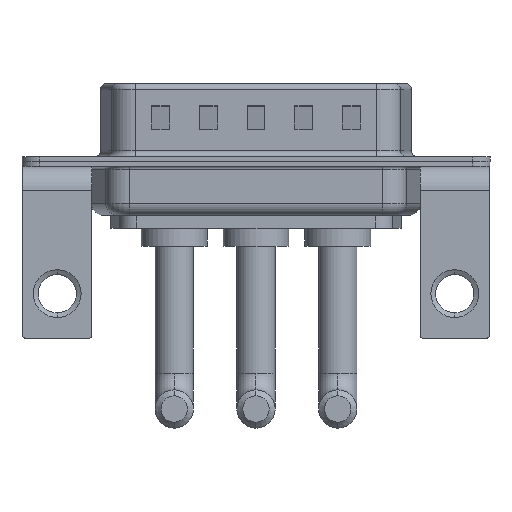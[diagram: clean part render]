
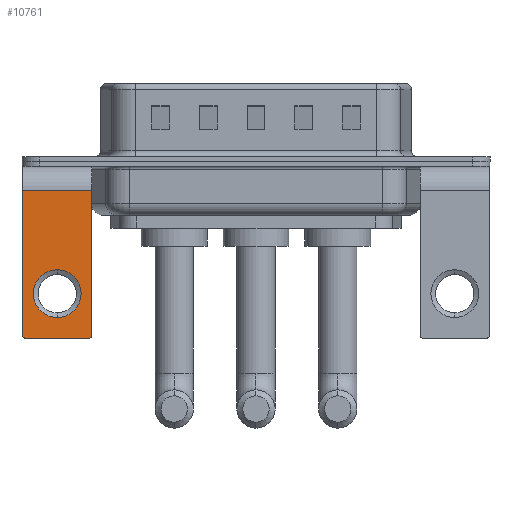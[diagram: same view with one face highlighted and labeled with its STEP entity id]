
A CAD part, front view. The second image highlights one B-rep face of the part: STEP entity #10761.
In plain terms, the highlighted planar face has unit normal (0, -1, 0).
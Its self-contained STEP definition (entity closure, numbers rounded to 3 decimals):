
#5 = DIRECTION ( 'NONE',  ( 0., -1., 0. ) ) ;
#497 = ORIENTED_EDGE ( 'NONE', *, *, #15092, .T. ) ;
#1039 = VERTEX_POINT ( 'NONE', #6492 ) ;
#1051 = VERTEX_POINT ( 'NONE', #1114 ) ;
#1114 = CARTESIAN_POINT ( 'NONE',  ( 2.65, -6.25, -14.8 ) ) ;
#1489 = LINE ( 'NONE', #6902, #2983 ) ;
#1558 = DIRECTION ( 'NONE',  ( 0., 1., 0. ) ) ;
#2467 = ORIENTED_EDGE ( 'NONE', *, *, #14313, .T. ) ;
#2516 = ORIENTED_EDGE ( 'NONE', *, *, #6081, .T. ) ;
#2701 = CIRCLE ( 'NONE', #8029, 0.25 ) ;
#2983 = VECTOR ( 'NONE', #9308, 1000. ) ;
#3414 = VECTOR ( 'NONE', #10062, 1000. ) ;
#3502 = VERTEX_POINT ( 'NONE', #15788 ) ;
#3541 = ORIENTED_EDGE ( 'NONE', *, *, #6380, .F. ) ;
#3632 = LINE ( 'NONE', #4635, #3414 ) ;
#3835 = AXIS2_PLACEMENT_3D ( 'NONE', #10567, #1558, #14381 ) ;
#4635 = CARTESIAN_POINT ( 'NONE',  ( 2.9, -6.25, -14.8 ) ) ;
#4720 = CARTESIAN_POINT ( 'NONE',  ( -2.9, -6.25, -2.4 ) ) ;
#4820 = CARTESIAN_POINT ( 'NONE',  ( 0., -6.25, -9.07 ) ) ;
#4837 = CARTESIAN_POINT ( 'NONE',  ( -2.65, -6.25, -14.55 ) ) ;
#5074 = DIRECTION ( 'NONE',  ( 0., 0., 1. ) ) ;
#5121 = DIRECTION ( 'NONE',  ( -1., 0., 0. ) ) ;
#5194 = VERTEX_POINT ( 'NONE', #13440 ) ;
#5683 = EDGE_LOOP ( 'NONE', ( #497, #13129 ) ) ;
#6081 = EDGE_CURVE ( 'NONE', #1039, #9286, #2701, .T. ) ;
#6197 = DIRECTION ( 'NONE',  ( 0., 1., 0. ) ) ;
#6380 = EDGE_CURVE ( 'NONE', #3502, #12796, #1489, .T. ) ;
#6492 = CARTESIAN_POINT ( 'NONE',  ( -2.9, -6.25, -14.55 ) ) ;
#6531 = LINE ( 'NONE', #8870, #16117 ) ;
#6902 = CARTESIAN_POINT ( 'NONE',  ( 2.9, -6.25, -2.4 ) ) ;
#7742 = EDGE_CURVE ( 'NONE', #1051, #12796, #9892, .T. ) ;
#8029 = AXIS2_PLACEMENT_3D ( 'NONE', #4837, #11024, #11188 ) ;
#8523 = CARTESIAN_POINT ( 'NONE',  ( 2.9, -6.25, -14.55 ) ) ;
#8718 = CIRCLE ( 'NONE', #10886, 2. ) ;
#8870 = CARTESIAN_POINT ( 'NONE',  ( 2.9, -6.25, -2.4 ) ) ;
#9056 = CARTESIAN_POINT ( 'NONE',  ( -2.9, -6.25, -2.4 ) ) ;
#9098 = ORIENTED_EDGE ( 'NONE', *, *, #9179, .T. ) ;
#9143 = ORIENTED_EDGE ( 'NONE', *, *, #15800, .F. ) ;
#9179 = EDGE_CURVE ( 'NONE', #15873, #1039, #14479, .T. ) ;
#9286 = VERTEX_POINT ( 'NONE', #13313 ) ;
#9308 = DIRECTION ( 'NONE',  ( 0., 0., -1. ) ) ;
#9620 = AXIS2_PLACEMENT_3D ( 'NONE', #11427, #5, #5074 ) ;
#9775 = CIRCLE ( 'NONE', #11907, 2. ) ;
#9892 = CIRCLE ( 'NONE', #9620, 0.25 ) ;
#9915 = DIRECTION ( 'NONE',  ( 0., 1., 0. ) ) ;
#10062 = DIRECTION ( 'NONE',  ( -1., 0., 0. ) ) ;
#10484 = FACE_BOUND ( 'NONE', #5683, .T. ) ;
#10567 = CARTESIAN_POINT ( 'NONE',  ( 2.9, -6.25, -2.4 ) ) ;
#10654 = FACE_OUTER_BOUND ( 'NONE', #11698, .T. ) ;
#10761 = ADVANCED_FACE ( 'NONE', ( #10484, #10654 ), #12962, .F. ) ;
#10841 = ORIENTED_EDGE ( 'NONE', *, *, #7742, .T. ) ;
#10886 = AXIS2_PLACEMENT_3D ( 'NONE', #11058, #6197, #11299 ) ;
#11024 = DIRECTION ( 'NONE',  ( 0., -1., 0. ) ) ;
#11058 = CARTESIAN_POINT ( 'NONE',  ( 0., -6.25, -11.07 ) ) ;
#11188 = DIRECTION ( 'NONE',  ( 0., 0., 1. ) ) ;
#11299 = DIRECTION ( 'NONE',  ( 0., 0., 1. ) ) ;
#11427 = CARTESIAN_POINT ( 'NONE',  ( 2.65, -6.25, -14.55 ) ) ;
#11698 = EDGE_LOOP ( 'NONE', ( #9098, #2516, #9143, #10841, #3541, #2467 ) ) ;
#11907 = AXIS2_PLACEMENT_3D ( 'NONE', #16388, #9915, #13567 ) ;
#12796 = VERTEX_POINT ( 'NONE', #8523 ) ;
#12962 = PLANE ( 'NONE',  #3835 ) ;
#13108 = VECTOR ( 'NONE', #14397, 1000. ) ;
#13129 = ORIENTED_EDGE ( 'NONE', *, *, #16310, .T. ) ;
#13313 = CARTESIAN_POINT ( 'NONE',  ( -2.65, -6.25, -14.8 ) ) ;
#13440 = CARTESIAN_POINT ( 'NONE',  ( 0., -6.25, -13.07 ) ) ;
#13567 = DIRECTION ( 'NONE',  ( 0., 0., 1. ) ) ;
#14313 = EDGE_CURVE ( 'NONE', #3502, #15873, #6531, .T. ) ;
#14381 = DIRECTION ( 'NONE',  ( 0., 0., 1. ) ) ;
#14397 = DIRECTION ( 'NONE',  ( 0., 0., -1. ) ) ;
#14479 = LINE ( 'NONE', #9056, #13108 ) ;
#15045 = VERTEX_POINT ( 'NONE', #4820 ) ;
#15092 = EDGE_CURVE ( 'NONE', #5194, #15045, #9775, .T. ) ;
#15788 = CARTESIAN_POINT ( 'NONE',  ( 2.9, -6.25, -2.4 ) ) ;
#15800 = EDGE_CURVE ( 'NONE', #1051, #9286, #3632, .T. ) ;
#15873 = VERTEX_POINT ( 'NONE', #4720 ) ;
#16117 = VECTOR ( 'NONE', #5121, 1000. ) ;
#16310 = EDGE_CURVE ( 'NONE', #15045, #5194, #8718, .T. ) ;
#16388 = CARTESIAN_POINT ( 'NONE',  ( 0., -6.25, -11.07 ) ) ;
